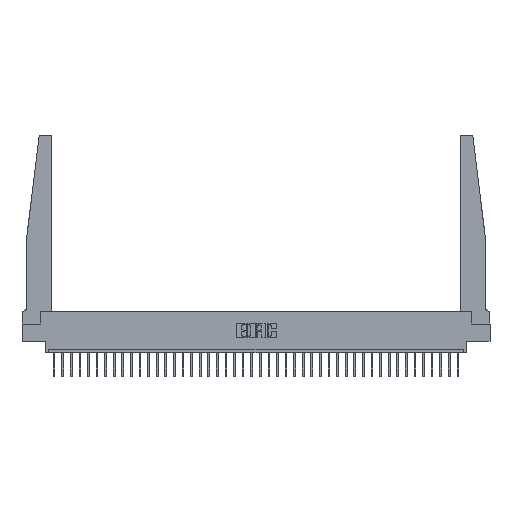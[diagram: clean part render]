
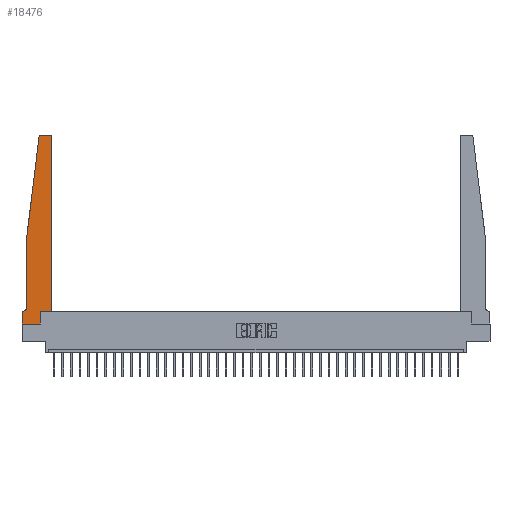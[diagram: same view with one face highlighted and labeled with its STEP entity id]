
A CAD part, top view. The second image highlights one B-rep face of the part: STEP entity #18476.
In plain terms, the highlighted planar face has unit normal (0, 0, 1).
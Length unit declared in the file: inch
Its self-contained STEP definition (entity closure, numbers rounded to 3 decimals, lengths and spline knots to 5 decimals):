
#734 = DIRECTION ( 'NONE',  ( 0., 0., 1. ) ) ;
#873 = CARTESIAN_POINT ( 'NONE',  ( 0.425, 2.72, 0.37 ) ) ;
#1457 = DIRECTION ( 'NONE',  ( 0., 0., 1. ) ) ;
#1525 = VECTOR ( 'NONE', #32537, 39.37008 ) ;
#1699 = LINE ( 'NONE', #19935, #16101 ) ;
#2070 = LINE ( 'NONE', #20001, #2507 ) ;
#2507 = VECTOR ( 'NONE', #26133, 39.37008 ) ;
#2540 = LINE ( 'NONE', #14873, #3813 ) ;
#2618 = ORIENTED_EDGE ( 'NONE', *, *, #28525, .T. ) ;
#2646 = VERTEX_POINT ( 'NONE', #21609 ) ;
#3193 = CIRCLE ( 'NONE', #12114, 0.05 ) ;
#3254 = ORIENTED_EDGE ( 'NONE', *, *, #23680, .T. ) ;
#3813 = VECTOR ( 'NONE', #17517, 39.37008 ) ;
#3934 = CARTESIAN_POINT ( 'NONE',  ( 0.27653, 2.75, 0.37 ) ) ;
#4406 = VERTEX_POINT ( 'NONE', #19079 ) ;
#5102 = ORIENTED_EDGE ( 'NONE', *, *, #33609, .T. ) ;
#5335 = VECTOR ( 'NONE', #7618, 39.37008 ) ;
#5957 = ORIENTED_EDGE ( 'NONE', *, *, #32022, .T. ) ;
#6169 = LINE ( 'NONE', #18509, #5335 ) ;
#6453 = VERTEX_POINT ( 'NONE', #17381 ) ;
#6718 = VERTEX_POINT ( 'NONE', #18242 ) ;
#7103 = EDGE_CURVE ( 'NONE', #10457, #24294, #1699, .T. ) ;
#7618 = DIRECTION ( 'NONE',  ( 0., -1., 0. ) ) ;
#7853 = EDGE_LOOP ( 'NONE', ( #5957, #18296, #5102, #25032, #3254, #2618, #29732, #19248, #16179, #16452, #10240, #30058 ) ) ;
#8240 = CARTESIAN_POINT ( 'NONE',  ( 0., 0.1875, 0.37 ) ) ;
#8544 = CARTESIAN_POINT ( 'NONE',  ( 0.395, 2.72, 0.37 ) ) ;
#8789 = AXIS2_PLACEMENT_3D ( 'NONE', #25200, #1457, #27825 ) ;
#8850 = EDGE_CURVE ( 'NONE', #23993, #10457, #6169, .T. ) ;
#9321 = DIRECTION ( 'NONE',  ( 1., 0., 0. ) ) ;
#9951 = VERTEX_POINT ( 'NONE', #18705 ) ;
#10240 = ORIENTED_EDGE ( 'NONE', *, *, #21862, .T. ) ;
#10285 = VERTEX_POINT ( 'NONE', #20175 ) ;
#10457 = VERTEX_POINT ( 'NONE', #26283 ) ;
#10544 = LINE ( 'NONE', #27289, #20843 ) ;
#11088 = CIRCLE ( 'NONE', #22132, 0.03 ) ;
#11638 = VERTEX_POINT ( 'NONE', #3934 ) ;
#12114 = AXIS2_PLACEMENT_3D ( 'NONE', #17422, #24961, #14557 ) ;
#13662 = DIRECTION ( 'NONE',  ( 1., 0., 0. ) ) ;
#13925 = PLANE ( 'NONE',  #23226 ) ;
#14035 = DIRECTION ( 'NONE',  ( 1., 0., 0. ) ) ;
#14143 = LINE ( 'NONE', #25433, #16619 ) ;
#14557 = DIRECTION ( 'NONE',  ( -1., 0., 0. ) ) ;
#14635 = CARTESIAN_POINT ( 'NONE',  ( 0.065, 0.1875, 0.37 ) ) ;
#14873 = CARTESIAN_POINT ( 'NONE',  ( 0.425, 0.18, 0.37 ) ) ;
#14955 = CIRCLE ( 'NONE', #8789, 0.03 ) ;
#16101 = VECTOR ( 'NONE', #18083, 39.37008 ) ;
#16179 = ORIENTED_EDGE ( 'NONE', *, *, #16982, .T. ) ;
#16452 = ORIENTED_EDGE ( 'NONE', *, *, #30885, .T. ) ;
#16574 = CARTESIAN_POINT ( 'NONE',  ( 0., 0.1875, 0.37 ) ) ;
#16619 = VECTOR ( 'NONE', #17438, 39.37008 ) ;
#16982 = EDGE_CURVE ( 'NONE', #24294, #6718, #2070, .T. ) ;
#17381 = CARTESIAN_POINT ( 'NONE',  ( 0.24675, 2.72367, 0.37 ) ) ;
#17422 = CARTESIAN_POINT ( 'NONE',  ( 0.015, 0.2375, 0.37 ) ) ;
#17438 = DIRECTION ( 'NONE',  ( -1., 0., 0. ) ) ;
#17517 = DIRECTION ( 'NONE',  ( 0., 1., 0. ) ) ;
#17577 = DIRECTION ( 'NONE',  ( 0., 0., 1. ) ) ;
#17886 = EDGE_CURVE ( 'NONE', #25184, #10285, #11088, .T. ) ;
#18083 = DIRECTION ( 'NONE',  ( 1., 0., 0. ) ) ;
#18242 = CARTESIAN_POINT ( 'NONE',  ( 0.2605, 0.18, 0.37 ) ) ;
#18296 = ORIENTED_EDGE ( 'NONE', *, *, #20697, .T. ) ;
#18476 = ADVANCED_FACE ( 'NONE', ( #20493 ), #13925, .T. ) ;
#18509 = CARTESIAN_POINT ( 'NONE',  ( 0., 0., 0.37 ) ) ;
#18705 = CARTESIAN_POINT ( 'NONE',  ( 0.065, 1.25, 0.37 ) ) ;
#19079 = CARTESIAN_POINT ( 'NONE',  ( 0.425, 0.18, 0.37 ) ) ;
#19248 = ORIENTED_EDGE ( 'NONE', *, *, #7103, .T. ) ;
#19935 = CARTESIAN_POINT ( 'NONE',  ( 0., 0., 0.37 ) ) ;
#20001 = CARTESIAN_POINT ( 'NONE',  ( 0.2605, 0.18, 0.37 ) ) ;
#20175 = CARTESIAN_POINT ( 'NONE',  ( 0.395, 2.75, 0.37 ) ) ;
#20214 = VECTOR ( 'NONE', #31612, 39.37008 ) ;
#20485 = LINE ( 'NONE', #14635, #1525 ) ;
#20493 = FACE_OUTER_BOUND ( 'NONE', #7853, .T. ) ;
#20697 = EDGE_CURVE ( 'NONE', #11638, #6453, #14955, .T. ) ;
#20843 = VECTOR ( 'NONE', #29802, 39.37008 ) ;
#21608 = CARTESIAN_POINT ( 'NONE',  ( 0.425, 0.18, 0.37 ) ) ;
#21609 = CARTESIAN_POINT ( 'NONE',  ( 0.065, 0.2375, 0.37 ) ) ;
#21862 = EDGE_CURVE ( 'NONE', #4406, #25184, #2540, .T. ) ;
#22132 = AXIS2_PLACEMENT_3D ( 'NONE', #8544, #734, #14035 ) ;
#23226 = AXIS2_PLACEMENT_3D ( 'NONE', #16574, #17577, #9321 ) ;
#23680 = EDGE_CURVE ( 'NONE', #2646, #28815, #3193, .T. ) ;
#23993 = VERTEX_POINT ( 'NONE', #8240 ) ;
#23998 = CARTESIAN_POINT ( 'NONE',  ( 0.065, 1.25, 0.37 ) ) ;
#24294 = VERTEX_POINT ( 'NONE', #33693 ) ;
#24961 = DIRECTION ( 'NONE',  ( 0., 0., -1. ) ) ;
#25032 = ORIENTED_EDGE ( 'NONE', *, *, #31028, .T. ) ;
#25184 = VERTEX_POINT ( 'NONE', #873 ) ;
#25200 = CARTESIAN_POINT ( 'NONE',  ( 0.27653, 2.72, 0.37 ) ) ;
#25433 = CARTESIAN_POINT ( 'NONE',  ( 0.25, 2.75, 0.37 ) ) ;
#25499 = LINE ( 'NONE', #23998, #20214 ) ;
#26119 = LINE ( 'NONE', #21608, #32223 ) ;
#26133 = DIRECTION ( 'NONE',  ( 0., 1., 0. ) ) ;
#26283 = CARTESIAN_POINT ( 'NONE',  ( 0., 0., 0.37 ) ) ;
#27289 = CARTESIAN_POINT ( 'NONE',  ( 0.065, 1.25, 0.37 ) ) ;
#27825 = DIRECTION ( 'NONE',  ( 1., 0., 0. ) ) ;
#28525 = EDGE_CURVE ( 'NONE', #28815, #23993, #20485, .T. ) ;
#28815 = VERTEX_POINT ( 'NONE', #33540 ) ;
#29732 = ORIENTED_EDGE ( 'NONE', *, *, #8850, .T. ) ;
#29802 = DIRECTION ( 'NONE',  ( 0., -1., 0. ) ) ;
#30058 = ORIENTED_EDGE ( 'NONE', *, *, #17886, .T. ) ;
#30885 = EDGE_CURVE ( 'NONE', #6718, #4406, #26119, .T. ) ;
#31028 = EDGE_CURVE ( 'NONE', #9951, #2646, #10544, .T. ) ;
#31612 = DIRECTION ( 'NONE',  ( -0.122, -0.992, 0. ) ) ;
#32022 = EDGE_CURVE ( 'NONE', #10285, #11638, #14143, .T. ) ;
#32223 = VECTOR ( 'NONE', #13662, 39.37008 ) ;
#32537 = DIRECTION ( 'NONE',  ( -1., 0., 0. ) ) ;
#33540 = CARTESIAN_POINT ( 'NONE',  ( 0.015, 0.1875, 0.37 ) ) ;
#33609 = EDGE_CURVE ( 'NONE', #6453, #9951, #25499, .T. ) ;
#33693 = CARTESIAN_POINT ( 'NONE',  ( 0.2605, 0., 0.37 ) ) ;
